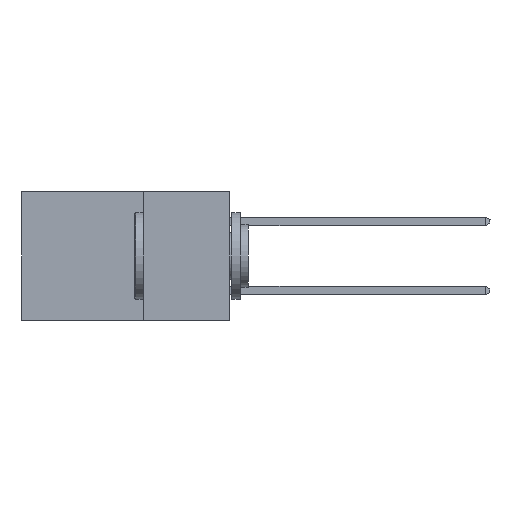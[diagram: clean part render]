
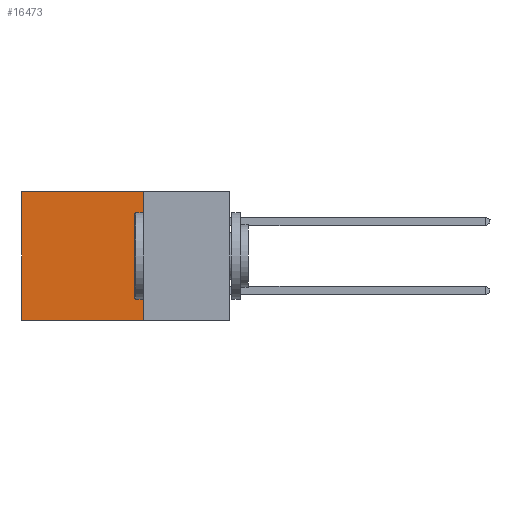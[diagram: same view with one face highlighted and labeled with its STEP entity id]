
A CAD part, left-side view. The second image highlights one B-rep face of the part: STEP entity #16473.
In plain terms, the highlighted planar face has unit normal (-1, 0, 0).
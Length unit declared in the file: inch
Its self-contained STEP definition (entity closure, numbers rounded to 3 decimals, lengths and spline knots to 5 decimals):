
#467 = LINE ( 'NONE', #17097, #11931 ) ;
#1809 = CARTESIAN_POINT ( 'NONE',  ( 0.298, 0.25, 0. ) ) ;
#1975 = DIRECTION ( 'NONE',  ( 0., 0., -1. ) ) ;
#2141 = DIRECTION ( 'NONE',  ( 0., 0., -1. ) ) ;
#2448 = CARTESIAN_POINT ( 'NONE',  ( 0.298, 0.25, -0.37 ) ) ;
#3742 = EDGE_CURVE ( 'NONE', #8617, #9363, #17101, .T. ) ;
#4491 = DIRECTION ( 'NONE',  ( 0., 1., 0. ) ) ;
#4880 = LINE ( 'NONE', #5298, #11454 ) ;
#5217 = VECTOR ( 'NONE', #5367, 39.37008 ) ;
#5298 = CARTESIAN_POINT ( 'NONE',  ( 0.298, 0.25, 0. ) ) ;
#5316 = VERTEX_POINT ( 'NONE', #17388 ) ;
#5367 = DIRECTION ( 'NONE',  ( 0., 0., -1. ) ) ;
#6286 = EDGE_CURVE ( 'NONE', #12546, #5316, #4880, .T. ) ;
#6991 = ORIENTED_EDGE ( 'NONE', *, *, #3742, .T. ) ;
#7285 = FACE_OUTER_BOUND ( 'NONE', #8972, .T. ) ;
#8617 = VERTEX_POINT ( 'NONE', #18204 ) ;
#8972 = EDGE_LOOP ( 'NONE', ( #6991, #11583, #13913, #13435 ) ) ;
#9363 = VERTEX_POINT ( 'NONE', #20071 ) ;
#9825 = EDGE_CURVE ( 'NONE', #12546, #8617, #467, .T. ) ;
#10137 = DIRECTION ( 'NONE',  ( 0., 1., 0. ) ) ;
#11454 = VECTOR ( 'NONE', #2141, 39.37008 ) ;
#11583 = ORIENTED_EDGE ( 'NONE', *, *, #16693, .F. ) ;
#11652 = LINE ( 'NONE', #2448, #17942 ) ;
#11931 = VECTOR ( 'NONE', #4491, 39.37008 ) ;
#12546 = VERTEX_POINT ( 'NONE', #1809 ) ;
#12853 = DIRECTION ( 'NONE',  ( 1., 0., 0. ) ) ;
#13435 = ORIENTED_EDGE ( 'NONE', *, *, #9825, .T. ) ;
#13913 = ORIENTED_EDGE ( 'NONE', *, *, #6286, .F. ) ;
#13934 = CARTESIAN_POINT ( 'NONE',  ( 0.298, 0.25, 0. ) ) ;
#16328 = CARTESIAN_POINT ( 'NONE',  ( 0.298, 0.6, 0. ) ) ;
#16473 = ADVANCED_FACE ( 'NONE', ( #7285 ), #20045, .F. ) ;
#16693 = EDGE_CURVE ( 'NONE', #5316, #9363, #11652, .T. ) ;
#17097 = CARTESIAN_POINT ( 'NONE',  ( 0.298, 0.25, 0. ) ) ;
#17101 = LINE ( 'NONE', #16328, #5217 ) ;
#17388 = CARTESIAN_POINT ( 'NONE',  ( 0.298, 0.25, -0.37 ) ) ;
#17942 = VECTOR ( 'NONE', #10137, 39.37008 ) ;
#18204 = CARTESIAN_POINT ( 'NONE',  ( 0.298, 0.6, 0. ) ) ;
#19487 = AXIS2_PLACEMENT_3D ( 'NONE', #13934, #12853, #1975 ) ;
#20045 = PLANE ( 'NONE',  #19487 ) ;
#20071 = CARTESIAN_POINT ( 'NONE',  ( 0.298, 0.6, -0.37 ) ) ;
